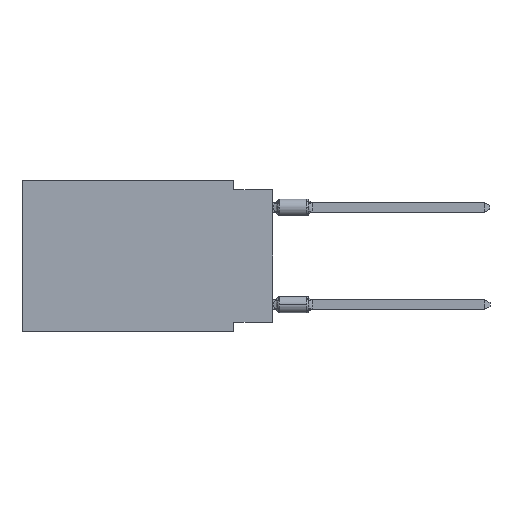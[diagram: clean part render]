
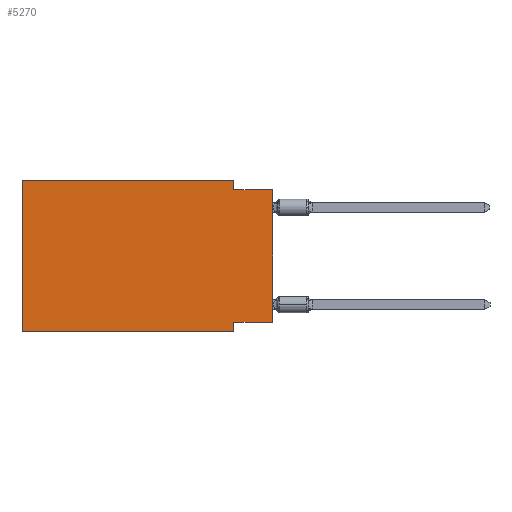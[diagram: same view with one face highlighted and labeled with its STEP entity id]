
A CAD part, left-side view. The second image highlights one B-rep face of the part: STEP entity #5270.
In plain terms, the highlighted planar face has unit normal (-1, 0, 0).
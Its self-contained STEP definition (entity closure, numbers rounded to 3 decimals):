
#254 = DIRECTION ( 'NONE',  ( 0., 1., 0. ) ) ;
#461 = ORIENTED_EDGE ( 'NONE', *, *, #8905, .F. ) ;
#588 = CARTESIAN_POINT ( 'NONE',  ( 0., 16.383, -9.906 ) ) ;
#699 = VERTEX_POINT ( 'NONE', #9806 ) ;
#875 = VERTEX_POINT ( 'NONE', #8857 ) ;
#1116 = VECTOR ( 'NONE', #14356, 1000. ) ;
#1907 = LINE ( 'NONE', #588, #15656 ) ;
#2066 = DIRECTION ( 'NONE',  ( 0., -1., 0. ) ) ;
#2280 = VERTEX_POINT ( 'NONE', #9134 ) ;
#2405 = VERTEX_POINT ( 'NONE', #11022 ) ;
#2477 = CARTESIAN_POINT ( 'NONE',  ( 0., 0., -0.635 ) ) ;
#2904 = CARTESIAN_POINT ( 'NONE',  ( 0., 2.54, 0. ) ) ;
#3754 = CARTESIAN_POINT ( 'NONE',  ( 0., 2.54, 0. ) ) ;
#4066 = LINE ( 'NONE', #2477, #10073 ) ;
#5143 = VECTOR ( 'NONE', #18045, 1000. ) ;
#5270 = ADVANCED_FACE ( 'NONE', ( #6886 ), #12591, .F. ) ;
#5338 = AXIS2_PLACEMENT_3D ( 'NONE', #18315, #8732, #10148 ) ;
#5575 = DIRECTION ( 'NONE',  ( 0., -1., 0. ) ) ;
#5831 = EDGE_LOOP ( 'NONE', ( #11217, #12304, #12116, #18490, #15288, #15707, #9454, #461 ) ) ;
#5958 = DIRECTION ( 'NONE',  ( 0., -1., 0. ) ) ;
#6488 = LINE ( 'NONE', #9382, #9685 ) ;
#6886 = FACE_OUTER_BOUND ( 'NONE', #5831, .T. ) ;
#6984 = VERTEX_POINT ( 'NONE', #3754 ) ;
#7192 = EDGE_CURVE ( 'NONE', #6984, #12882, #8636, .T. ) ;
#8636 = LINE ( 'NONE', #2904, #1116 ) ;
#8732 = DIRECTION ( 'NONE',  ( 1., 0., 0. ) ) ;
#8801 = LINE ( 'NONE', #9773, #12140 ) ;
#8857 = CARTESIAN_POINT ( 'NONE',  ( 0., 0., -0.635 ) ) ;
#8905 = EDGE_CURVE ( 'NONE', #14108, #2280, #8801, .T. ) ;
#9134 = CARTESIAN_POINT ( 'NONE',  ( 0., 2.54, -9.271 ) ) ;
#9227 = LINE ( 'NONE', #12226, #5143 ) ;
#9382 = CARTESIAN_POINT ( 'NONE',  ( 0., 16.383, 0. ) ) ;
#9454 = ORIENTED_EDGE ( 'NONE', *, *, #14915, .F. ) ;
#9495 = EDGE_CURVE ( 'NONE', #12882, #875, #4066, .T. ) ;
#9685 = VECTOR ( 'NONE', #2066, 1000. ) ;
#9773 = CARTESIAN_POINT ( 'NONE',  ( 0., 0., -9.271 ) ) ;
#9806 = CARTESIAN_POINT ( 'NONE',  ( 0., 2.54, -9.906 ) ) ;
#10073 = VECTOR ( 'NONE', #5575, 1000. ) ;
#10148 = DIRECTION ( 'NONE',  ( 0., 0., -1. ) ) ;
#10806 = CARTESIAN_POINT ( 'NONE',  ( 0., 16.383, -9.906 ) ) ;
#10889 = CARTESIAN_POINT ( 'NONE',  ( 0., 0., -9.271 ) ) ;
#11005 = LINE ( 'NONE', #14180, #14205 ) ;
#11022 = CARTESIAN_POINT ( 'NONE',  ( 0., 16.383, 0. ) ) ;
#11024 = CARTESIAN_POINT ( 'NONE',  ( 0., 16.383, 0. ) ) ;
#11217 = ORIENTED_EDGE ( 'NONE', *, *, #13289, .T. ) ;
#12116 = ORIENTED_EDGE ( 'NONE', *, *, #7192, .F. ) ;
#12140 = VECTOR ( 'NONE', #254, 1000. ) ;
#12166 = VECTOR ( 'NONE', #15420, 1000. ) ;
#12226 = CARTESIAN_POINT ( 'NONE',  ( 0., 2.54, -9.906 ) ) ;
#12304 = ORIENTED_EDGE ( 'NONE', *, *, #9495, .F. ) ;
#12591 = PLANE ( 'NONE',  #5338 ) ;
#12882 = VERTEX_POINT ( 'NONE', #15181 ) ;
#13289 = EDGE_CURVE ( 'NONE', #14108, #875, #11005, .T. ) ;
#13920 = LINE ( 'NONE', #11024, #12166 ) ;
#14105 = EDGE_CURVE ( 'NONE', #2405, #6984, #6488, .T. ) ;
#14108 = VERTEX_POINT ( 'NONE', #10889 ) ;
#14180 = CARTESIAN_POINT ( 'NONE',  ( 0., 0., 0. ) ) ;
#14205 = VECTOR ( 'NONE', #18406, 1000. ) ;
#14356 = DIRECTION ( 'NONE',  ( 0., 0., -1. ) ) ;
#14752 = EDGE_CURVE ( 'NONE', #16663, #699, #1907, .T. ) ;
#14915 = EDGE_CURVE ( 'NONE', #2280, #699, #9227, .T. ) ;
#15181 = CARTESIAN_POINT ( 'NONE',  ( 0., 2.54, -0.635 ) ) ;
#15288 = ORIENTED_EDGE ( 'NONE', *, *, #18093, .F. ) ;
#15420 = DIRECTION ( 'NONE',  ( 0., 0., 1. ) ) ;
#15656 = VECTOR ( 'NONE', #5958, 1000. ) ;
#15707 = ORIENTED_EDGE ( 'NONE', *, *, #14752, .T. ) ;
#16663 = VERTEX_POINT ( 'NONE', #10806 ) ;
#18045 = DIRECTION ( 'NONE',  ( 0., 0., -1. ) ) ;
#18093 = EDGE_CURVE ( 'NONE', #16663, #2405, #13920, .T. ) ;
#18315 = CARTESIAN_POINT ( 'NONE',  ( 0., 16.383, 0. ) ) ;
#18406 = DIRECTION ( 'NONE',  ( 0., 0., 1. ) ) ;
#18490 = ORIENTED_EDGE ( 'NONE', *, *, #14105, .F. ) ;
